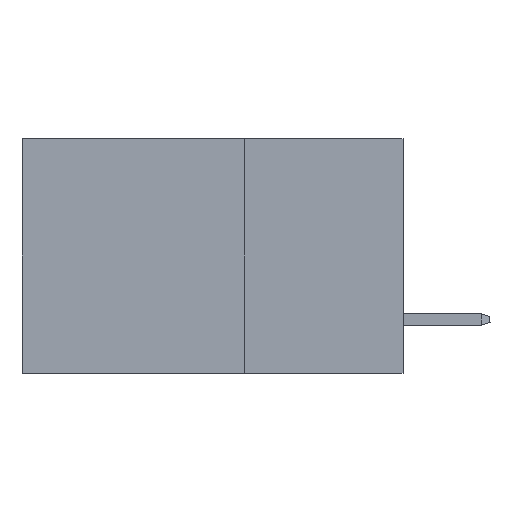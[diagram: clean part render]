
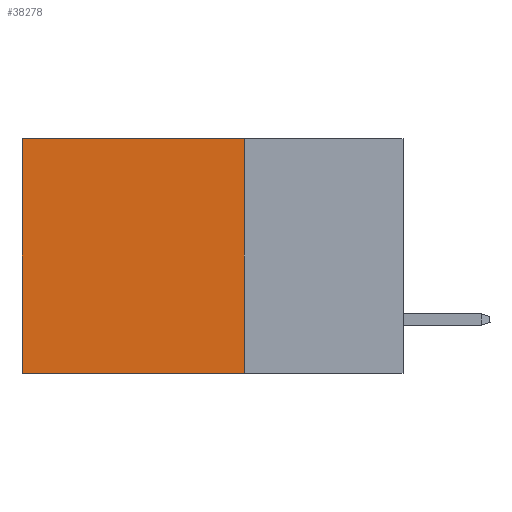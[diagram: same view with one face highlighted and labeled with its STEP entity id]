
A CAD part, left-side view. The second image highlights one B-rep face of the part: STEP entity #38278.
In plain terms, the highlighted planar face has unit normal (-1, 0, 0).
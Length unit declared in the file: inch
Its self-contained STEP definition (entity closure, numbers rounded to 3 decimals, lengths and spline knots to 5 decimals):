
#353 = ORIENTED_EDGE ( 'NONE', *, *, #32315, .T. ) ;
#1265 = ORIENTED_EDGE ( 'NONE', *, *, #27260, .F. ) ;
#2194 = DIRECTION ( 'NONE',  ( 0., 0., -1. ) ) ;
#4506 = LINE ( 'NONE', #41987, #10565 ) ;
#4750 = VECTOR ( 'NONE', #17147, 39.37008 ) ;
#4831 = CARTESIAN_POINT ( 'NONE',  ( 0.2875, 0.25, -0.37 ) ) ;
#5707 = LINE ( 'NONE', #22353, #11821 ) ;
#7253 = VERTEX_POINT ( 'NONE', #9385 ) ;
#7626 = VERTEX_POINT ( 'NONE', #12389 ) ;
#9385 = CARTESIAN_POINT ( 'NONE',  ( 0.2875, 0.6, -0.37 ) ) ;
#10068 = VERTEX_POINT ( 'NONE', #4831 ) ;
#10565 = VECTOR ( 'NONE', #25512, 39.37008 ) ;
#10991 = CARTESIAN_POINT ( 'NONE',  ( 0.2875, 0.25, 0. ) ) ;
#11574 = EDGE_CURVE ( 'NONE', #7626, #7253, #5707, .T. ) ;
#11821 = VECTOR ( 'NONE', #2194, 39.37008 ) ;
#11896 = ORIENTED_EDGE ( 'NONE', *, *, #40728, .F. ) ;
#12353 = DIRECTION ( 'NONE',  ( 1., 0., 0. ) ) ;
#12389 = CARTESIAN_POINT ( 'NONE',  ( 0.2875, 0.6, 0. ) ) ;
#12583 = VERTEX_POINT ( 'NONE', #10991 ) ;
#15643 = FACE_OUTER_BOUND ( 'NONE', #21044, .T. ) ;
#16231 = DIRECTION ( 'NONE',  ( 0., 0., -1. ) ) ;
#17147 = DIRECTION ( 'NONE',  ( 0., 1., 0. ) ) ;
#18813 = AXIS2_PLACEMENT_3D ( 'NONE', #42867, #12353, #30548 ) ;
#21044 = EDGE_LOOP ( 'NONE', ( #41190, #1265, #11896, #353 ) ) ;
#22353 = CARTESIAN_POINT ( 'NONE',  ( 0.2875, 0.6, 0. ) ) ;
#25512 = DIRECTION ( 'NONE',  ( 0., 1., 0. ) ) ;
#27260 = EDGE_CURVE ( 'NONE', #10068, #7253, #28563, .T. ) ;
#28563 = LINE ( 'NONE', #42861, #4750 ) ;
#29604 = LINE ( 'NONE', #36203, #30102 ) ;
#30102 = VECTOR ( 'NONE', #16231, 39.37008 ) ;
#30548 = DIRECTION ( 'NONE',  ( 0., 0., -1. ) ) ;
#32315 = EDGE_CURVE ( 'NONE', #12583, #7626, #4506, .T. ) ;
#36203 = CARTESIAN_POINT ( 'NONE',  ( 0.2875, 0.25, 0. ) ) ;
#38278 = ADVANCED_FACE ( 'NONE', ( #15643 ), #42425, .F. ) ;
#40728 = EDGE_CURVE ( 'NONE', #12583, #10068, #29604, .T. ) ;
#41190 = ORIENTED_EDGE ( 'NONE', *, *, #11574, .T. ) ;
#41987 = CARTESIAN_POINT ( 'NONE',  ( 0.2875, 0.25, 0. ) ) ;
#42425 = PLANE ( 'NONE',  #18813 ) ;
#42861 = CARTESIAN_POINT ( 'NONE',  ( 0.2875, 0.25, -0.37 ) ) ;
#42867 = CARTESIAN_POINT ( 'NONE',  ( 0.2875, 0.25, 0. ) ) ;
